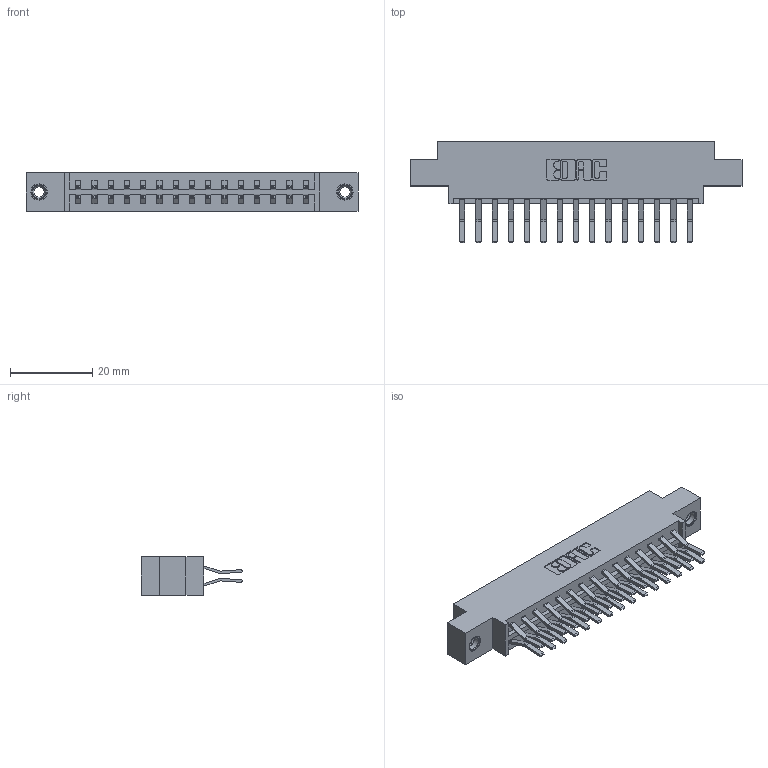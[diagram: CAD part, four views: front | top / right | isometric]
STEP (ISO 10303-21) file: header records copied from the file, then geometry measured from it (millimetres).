
FILE_DESCRIPTION (( 'STEP AP203' ), '1' );
FILE_NAME ('333-030-560-807.STEP', '2018-08-02T19:04:24', ( '' ), ( '' ), 'SwSTEP 2.0', 'SolidWorks 2016', '' );
FILE_SCHEMA (( 'CONFIG_CONTROL_DESIGN' ));
Length unit declared in the file: inch
Products named in the file (4): 345-250-001_345-250-005-103; 333-030-560-807; 345-292-001_560 Tail; 333 Part_Offset - .156 Dia - TI
Assembly tree (33 placements, depth 2):
  333-030-560-807
    333 Part_Offset - .156 Dia - TI
    345-292-001_560 Tail  x30
    345-250-001_345-250-005-103  x2
Bounding box: 80.98 x 24.78 x 9.4 mm (x, y, z)
Volume: 7969.9 mm3; surface area: 9948.2 mm2
Topology: 33 solids, 33 shells, 1798 faces, 5289 edges, 3478 vertices
Faces by surface type: plane 1186, cylinder 596, cone 12, torus 4
Entity records: 14548 total; most frequent: CARTESIAN_POINT 2429, ORIENTED_EDGE 2358, DIRECTION 2157, EDGE_CURVE 1179, LINE 1027, VECTOR 1027, VERTEX_POINT 780, AXIS2_PLACEMENT_3D 565
